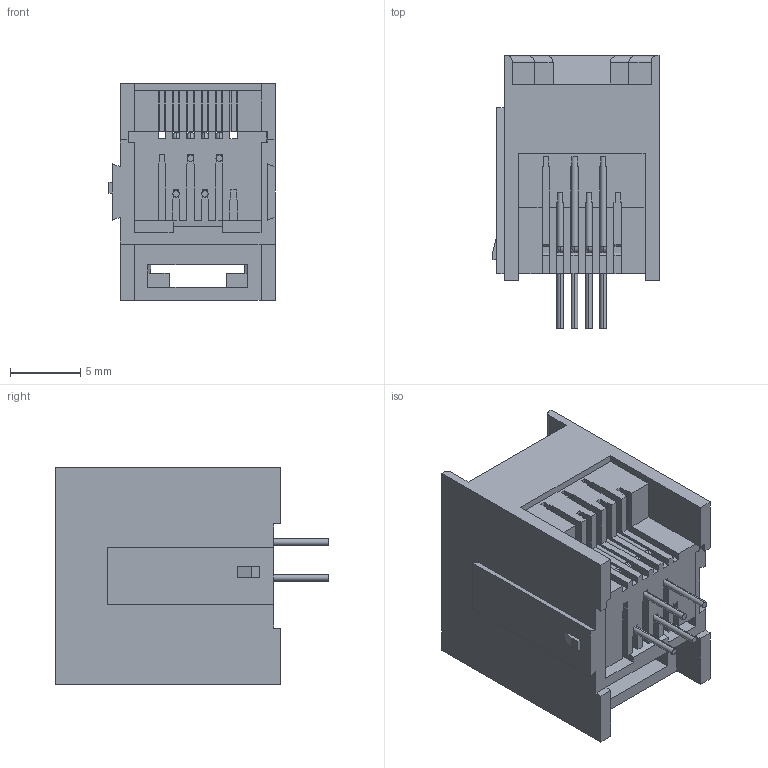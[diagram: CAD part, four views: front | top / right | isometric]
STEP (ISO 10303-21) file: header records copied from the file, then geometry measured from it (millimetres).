
FILE_DESCRIPTION (( 'STEP AP203' ), '1' );
FILE_NAME ('J2X016491P00030.STEP', '2020-07-29T15:02:57', ( '' ), ( '' ), 'SwSTEP 2.0', 'SolidWorks 2020', '' );
FILE_SCHEMA (( 'CONFIG_CONTROL_DESIGN' ));
Length unit declared in the file: millimetre
Products named in the file (4): 2X Contacts_6P4C; J2X016491P00030; 2X Contact Lock; 2X Insulator
Assembly tree (3 placements, depth 2):
  J2X016491P00030
    2X Insulator
    2X Contacts_6P4C
    2X Contact Lock
Bounding box: 11.81 x 19.4 x 15.4 mm (x, y, z)
Volume: 1209.7 mm3; surface area: 2765.8 mm2
Topology: 6 solids, 6 shells, 434 faces, 1289 edges, 833 vertices
Faces by surface type: plane 329, cylinder 81, bspline 24
Entity records: 15365 total; most frequent: CARTESIAN_POINT 3368, ORIENTED_EDGE 2546, DIRECTION 2279, EDGE_CURVE 1273, LINE 1059, VECTOR 1059, VERTEX_POINT 833, AXIS2_PLACEMENT_3D 610
